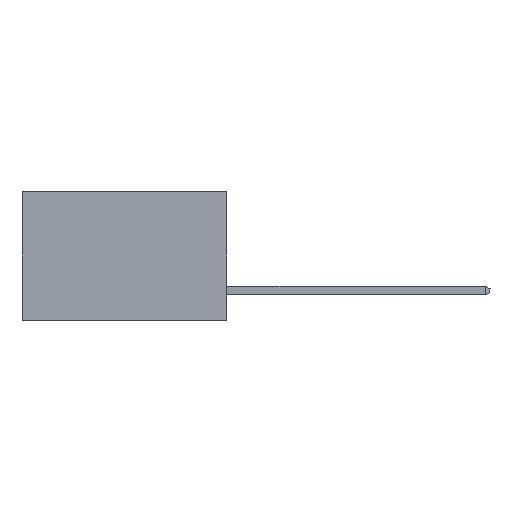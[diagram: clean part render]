
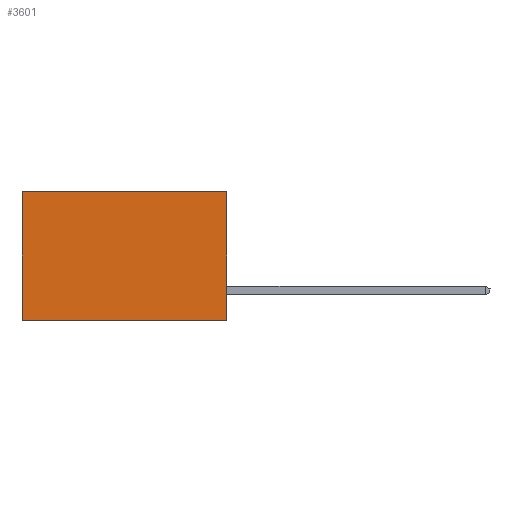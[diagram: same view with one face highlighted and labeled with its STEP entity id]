
A CAD part, left-side view. The second image highlights one B-rep face of the part: STEP entity #3601.
In plain terms, the highlighted planar face has unit normal (-1, 0, 0).
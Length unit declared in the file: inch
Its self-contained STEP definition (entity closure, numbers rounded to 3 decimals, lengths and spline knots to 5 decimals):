
#109 = VERTEX_POINT ( 'NONE', #3368 ) ;
#150 = FACE_OUTER_BOUND ( 'NONE', #2258, .T. ) ;
#478 = ORIENTED_EDGE ( 'NONE', *, *, #2419, .T. ) ;
#528 = LINE ( 'NONE', #3435, #5037 ) ;
#597 = ORIENTED_EDGE ( 'NONE', *, *, #6745, .F. ) ;
#1120 = VECTOR ( 'NONE', #3193, 39.37008 ) ;
#1411 = ORIENTED_EDGE ( 'NONE', *, *, #6703, .F. ) ;
#1775 = DIRECTION ( 'NONE',  ( 0., 0., -1. ) ) ;
#1882 = CARTESIAN_POINT ( 'NONE',  ( 0.277, 0., -0.37 ) ) ;
#1914 = CARTESIAN_POINT ( 'NONE',  ( 0.277, 0., -0.37 ) ) ;
#2258 = EDGE_LOOP ( 'NONE', ( #478, #1411, #597, #4423 ) ) ;
#2276 = VERTEX_POINT ( 'NONE', #3886 ) ;
#2404 = DIRECTION ( 'NONE',  ( 1., 0., 0. ) ) ;
#2419 = EDGE_CURVE ( 'NONE', #3353, #2276, #7025, .T. ) ;
#2448 = CARTESIAN_POINT ( 'NONE',  ( 0.277, 0., -0.37 ) ) ;
#2885 = VECTOR ( 'NONE', #1775, 39.37008 ) ;
#3108 = DIRECTION ( 'NONE',  ( 0., 1., 0. ) ) ;
#3193 = DIRECTION ( 'NONE',  ( 0., 0., -1. ) ) ;
#3291 = DIRECTION ( 'NONE',  ( 0., 1., 0. ) ) ;
#3353 = VERTEX_POINT ( 'NONE', #4027 ) ;
#3368 = CARTESIAN_POINT ( 'NONE',  ( 0.277, 0., 0. ) ) ;
#3435 = CARTESIAN_POINT ( 'NONE',  ( 0.277, 0., -0.37 ) ) ;
#3463 = LINE ( 'NONE', #6165, #4866 ) ;
#3601 = ADVANCED_FACE ( 'NONE', ( #150 ), #6110, .F. ) ;
#3886 = CARTESIAN_POINT ( 'NONE',  ( 0.277, 0.59, -0.37 ) ) ;
#3930 = AXIS2_PLACEMENT_3D ( 'NONE', #1882, #2404, #4993 ) ;
#4027 = CARTESIAN_POINT ( 'NONE',  ( 0.277, 0.59, 0. ) ) ;
#4236 = CARTESIAN_POINT ( 'NONE',  ( 0.277, 0.59, -0.37 ) ) ;
#4342 = VERTEX_POINT ( 'NONE', #2448 ) ;
#4423 = ORIENTED_EDGE ( 'NONE', *, *, #6915, .T. ) ;
#4866 = VECTOR ( 'NONE', #3291, 39.37008 ) ;
#4993 = DIRECTION ( 'NONE',  ( 0., 0., -1. ) ) ;
#5037 = VECTOR ( 'NONE', #3108, 39.37008 ) ;
#6110 = PLANE ( 'NONE',  #3930 ) ;
#6165 = CARTESIAN_POINT ( 'NONE',  ( 0.277, 0., 0. ) ) ;
#6703 = EDGE_CURVE ( 'NONE', #4342, #2276, #528, .T. ) ;
#6745 = EDGE_CURVE ( 'NONE', #109, #4342, #7239, .T. ) ;
#6915 = EDGE_CURVE ( 'NONE', #109, #3353, #3463, .T. ) ;
#7025 = LINE ( 'NONE', #4236, #1120 ) ;
#7239 = LINE ( 'NONE', #1914, #2885 ) ;
